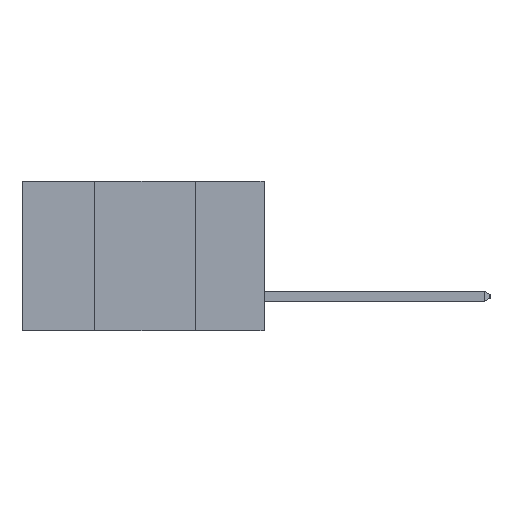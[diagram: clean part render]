
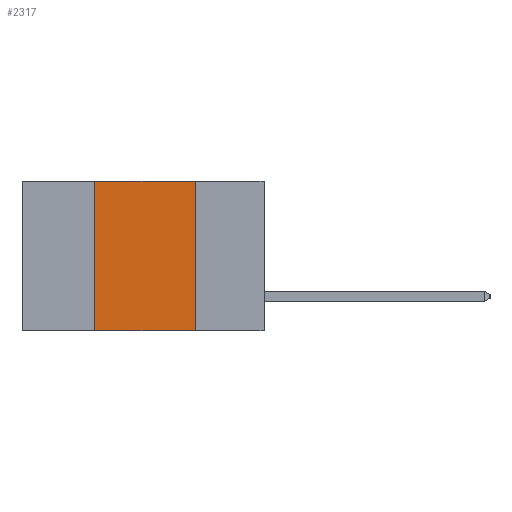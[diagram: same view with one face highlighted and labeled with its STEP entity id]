
A CAD part, left-side view. The second image highlights one B-rep face of the part: STEP entity #2317.
In plain terms, the highlighted planar face has unit normal (-1, 0, 0).
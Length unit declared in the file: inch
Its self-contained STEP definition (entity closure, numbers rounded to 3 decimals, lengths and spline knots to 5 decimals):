
#598 = LINE ( 'NONE', #6456, #9458 ) ;
#721 = DIRECTION ( 'NONE',  ( 0., 0., -1. ) ) ;
#744 = DIRECTION ( 'NONE',  ( 1., 0., 0. ) ) ;
#792 = PLANE ( 'NONE',  #9363 ) ;
#815 = CARTESIAN_POINT ( 'NONE',  ( 0., 0.6, 0. ) ) ;
#1318 = VERTEX_POINT ( 'NONE', #7601 ) ;
#1947 = CARTESIAN_POINT ( 'NONE',  ( 0., 0.6, 0. ) ) ;
#2212 = DIRECTION ( 'NONE',  ( 0., -1., 0. ) ) ;
#2317 = ADVANCED_FACE ( 'NONE', ( #6789 ), #792, .F. ) ;
#2696 = VECTOR ( 'NONE', #2212, 39.37008 ) ;
#3501 = VERTEX_POINT ( 'NONE', #7349 ) ;
#3920 = CARTESIAN_POINT ( 'NONE',  ( 0., 0.17, 0. ) ) ;
#3930 = CARTESIAN_POINT ( 'NONE',  ( 0., 0.6, -0.37 ) ) ;
#4563 = CARTESIAN_POINT ( 'NONE',  ( 0., 0.42, 0. ) ) ;
#4782 = ORIENTED_EDGE ( 'NONE', *, *, #7694, .F. ) ;
#5226 = LINE ( 'NONE', #3930, #2696 ) ;
#5368 = EDGE_CURVE ( 'NONE', #3501, #1318, #5226, .T. ) ;
#5534 = ORIENTED_EDGE ( 'NONE', *, *, #5368, .T. ) ;
#5625 = DIRECTION ( 'NONE',  ( 0., 0., -1. ) ) ;
#5627 = VECTOR ( 'NONE', #9765, 39.37008 ) ;
#5872 = VERTEX_POINT ( 'NONE', #4563 ) ;
#6222 = DIRECTION ( 'NONE',  ( 0., -1., 0. ) ) ;
#6456 = CARTESIAN_POINT ( 'NONE',  ( 0., 0.17, -0.37 ) ) ;
#6789 = FACE_OUTER_BOUND ( 'NONE', #9712, .T. ) ;
#7123 = EDGE_CURVE ( 'NONE', #3501, #5872, #10143, .T. ) ;
#7136 = ORIENTED_EDGE ( 'NONE', *, *, #7123, .F. ) ;
#7349 = CARTESIAN_POINT ( 'NONE',  ( 0., 0.42, -0.37 ) ) ;
#7601 = CARTESIAN_POINT ( 'NONE',  ( 0., 0.17, -0.37 ) ) ;
#7694 = EDGE_CURVE ( 'NONE', #5872, #8885, #9090, .T. ) ;
#8237 = EDGE_CURVE ( 'NONE', #8885, #1318, #598, .T. ) ;
#8885 = VERTEX_POINT ( 'NONE', #3920 ) ;
#9090 = LINE ( 'NONE', #1947, #10767 ) ;
#9363 = AXIS2_PLACEMENT_3D ( 'NONE', #815, #744, #721 ) ;
#9458 = VECTOR ( 'NONE', #5625, 39.37008 ) ;
#9712 = EDGE_LOOP ( 'NONE', ( #10753, #4782, #7136, #5534 ) ) ;
#9765 = DIRECTION ( 'NONE',  ( 0., 0., 1. ) ) ;
#10143 = LINE ( 'NONE', #10577, #5627 ) ;
#10577 = CARTESIAN_POINT ( 'NONE',  ( 0., 0.42, -0.37 ) ) ;
#10753 = ORIENTED_EDGE ( 'NONE', *, *, #8237, .F. ) ;
#10767 = VECTOR ( 'NONE', #6222, 39.37008 ) ;
